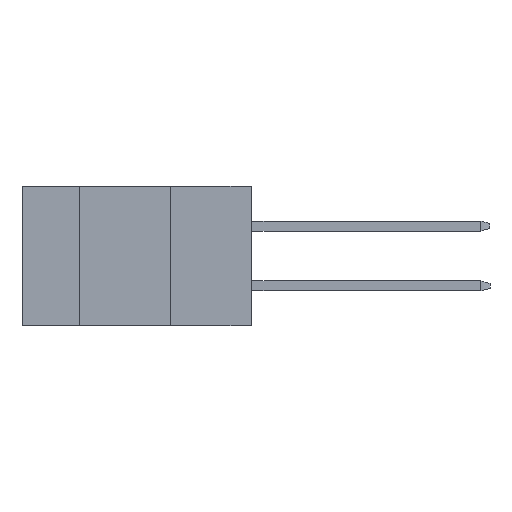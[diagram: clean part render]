
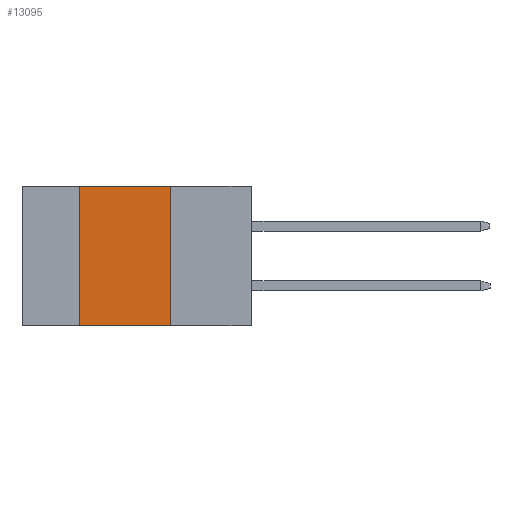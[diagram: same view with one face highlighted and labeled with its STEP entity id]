
A CAD part, left-side view. The second image highlights one B-rep face of the part: STEP entity #13095.
In plain terms, the highlighted planar face has unit normal (-1, 0, 0).
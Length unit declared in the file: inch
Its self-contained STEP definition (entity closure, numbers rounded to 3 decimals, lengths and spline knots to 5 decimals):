
#35 = ORIENTED_EDGE ( 'NONE', *, *, #17786, .F. ) ;
#466 = VECTOR ( 'NONE', #4091, 39.37008 ) ;
#558 = VECTOR ( 'NONE', #16650, 39.37008 ) ;
#796 = VERTEX_POINT ( 'NONE', #6479 ) ;
#799 = DIRECTION ( 'NONE',  ( 0., 0., 1. ) ) ;
#1793 = PLANE ( 'NONE',  #16341 ) ;
#3315 = FACE_OUTER_BOUND ( 'NONE', #13771, .T. ) ;
#3747 = DIRECTION ( 'NONE',  ( 0., -1., 0. ) ) ;
#3860 = LINE ( 'NONE', #15506, #558 ) ;
#4091 = DIRECTION ( 'NONE',  ( 0., -1., 0. ) ) ;
#4712 = CARTESIAN_POINT ( 'NONE',  ( 0., 0.254, -0.437 ) ) ;
#5291 = ORIENTED_EDGE ( 'NONE', *, *, #13759, .F. ) ;
#6479 = CARTESIAN_POINT ( 'NONE',  ( 0., 0.54, 0. ) ) ;
#7173 = CARTESIAN_POINT ( 'NONE',  ( 0., 0.254, 0. ) ) ;
#8383 = VERTEX_POINT ( 'NONE', #7173 ) ;
#8881 = ORIENTED_EDGE ( 'NONE', *, *, #11903, .F. ) ;
#9152 = CARTESIAN_POINT ( 'NONE',  ( 0., 0.72, 0. ) ) ;
#10945 = LINE ( 'NONE', #11034, #11803 ) ;
#11034 = CARTESIAN_POINT ( 'NONE',  ( 0., 0.72, 0. ) ) ;
#11803 = VECTOR ( 'NONE', #3747, 39.37008 ) ;
#11903 = EDGE_CURVE ( 'NONE', #15175, #796, #18284, .T. ) ;
#12281 = EDGE_CURVE ( 'NONE', #15175, #17672, #14211, .T. ) ;
#13095 = ADVANCED_FACE ( 'NONE', ( #3315 ), #1793, .F. ) ;
#13347 = DIRECTION ( 'NONE',  ( 1., 0., 0. ) ) ;
#13443 = DIRECTION ( 'NONE',  ( 0., 0., -1. ) ) ;
#13759 = EDGE_CURVE ( 'NONE', #796, #8383, #10945, .T. ) ;
#13771 = EDGE_LOOP ( 'NONE', ( #35, #5291, #8881, #16113 ) ) ;
#13879 = CARTESIAN_POINT ( 'NONE',  ( 0., 0.54, -0.437 ) ) ;
#14116 = CARTESIAN_POINT ( 'NONE',  ( 0., 0.72, -0.437 ) ) ;
#14211 = LINE ( 'NONE', #14116, #466 ) ;
#15175 = VERTEX_POINT ( 'NONE', #17753 ) ;
#15506 = CARTESIAN_POINT ( 'NONE',  ( 0., 0.254, -0.437 ) ) ;
#16113 = ORIENTED_EDGE ( 'NONE', *, *, #12281, .T. ) ;
#16341 = AXIS2_PLACEMENT_3D ( 'NONE', #9152, #13347, #13443 ) ;
#16650 = DIRECTION ( 'NONE',  ( 0., 0., -1. ) ) ;
#17672 = VERTEX_POINT ( 'NONE', #4712 ) ;
#17753 = CARTESIAN_POINT ( 'NONE',  ( 0., 0.54, -0.437 ) ) ;
#17786 = EDGE_CURVE ( 'NONE', #8383, #17672, #3860, .T. ) ;
#17854 = VECTOR ( 'NONE', #799, 39.37008 ) ;
#18284 = LINE ( 'NONE', #13879, #17854 ) ;
